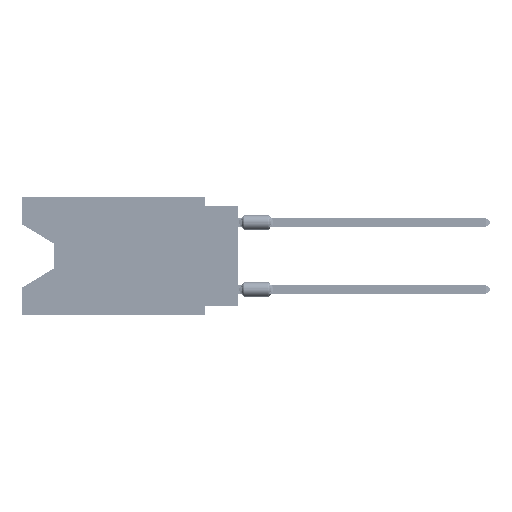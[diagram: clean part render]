
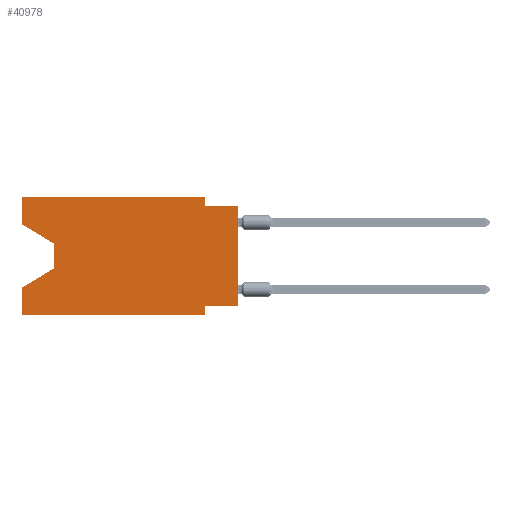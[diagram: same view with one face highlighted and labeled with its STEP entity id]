
A CAD part, left-side view. The second image highlights one B-rep face of the part: STEP entity #40978.
In plain terms, the highlighted planar face has unit normal (-1, 0, 0).
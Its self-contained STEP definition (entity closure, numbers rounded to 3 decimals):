
#410 = EDGE_CURVE ( 'NONE', #22969, #66952, #97227, .T. ) ;
#1054 = DIRECTION ( 'NONE',  ( 0., 0., -1. ) ) ;
#1590 = LINE ( 'NONE', #68167, #106151 ) ;
#3499 = ORIENTED_EDGE ( 'NONE', *, *, #56066, .T. ) ;
#3960 = DIRECTION ( 'NONE',  ( 0., 0., -1. ) ) ;
#5031 = PLANE ( 'NONE',  #49814 ) ;
#7524 = CARTESIAN_POINT ( 'NONE',  ( 0., 2.54, -0.635 ) ) ;
#9177 = VERTEX_POINT ( 'NONE', #7524 ) ;
#12287 = CARTESIAN_POINT ( 'NONE',  ( 0., 13.97, -3.505 ) ) ;
#13808 = CARTESIAN_POINT ( 'NONE',  ( 0., 2.54, -8.255 ) ) ;
#14338 = DIRECTION ( 'NONE',  ( 0., 0.855, -0.519 ) ) ;
#14988 = CARTESIAN_POINT ( 'NONE',  ( 0., 2.54, 0. ) ) ;
#15196 = VERTEX_POINT ( 'NONE', #34974 ) ;
#17138 = DIRECTION ( 'NONE',  ( 0., 0., 1. ) ) ;
#17782 = DIRECTION ( 'NONE',  ( 0., 0., 1. ) ) ;
#19921 = ORIENTED_EDGE ( 'NONE', *, *, #41716, .F. ) ;
#20324 = FACE_OUTER_BOUND ( 'NONE', #63549, .T. ) ;
#22209 = EDGE_CURVE ( 'NONE', #15196, #106065, #46941, .T. ) ;
#22969 = VERTEX_POINT ( 'NONE', #81820 ) ;
#23919 = DIRECTION ( 'NONE',  ( 0., -1., 0. ) ) ;
#24839 = EDGE_CURVE ( 'NONE', #106065, #89694, #95804, .T. ) ;
#25006 = LINE ( 'NONE', #98647, #97730 ) ;
#25774 = ORIENTED_EDGE ( 'NONE', *, *, #36053, .T. ) ;
#27647 = DIRECTION ( 'NONE',  ( 0., -1., 0. ) ) ;
#28692 = VERTEX_POINT ( 'NONE', #44951 ) ;
#29619 = CARTESIAN_POINT ( 'NONE',  ( 0., 16.383, 0. ) ) ;
#29656 = CARTESIAN_POINT ( 'NONE',  ( 0., 13.97, -3.505 ) ) ;
#29750 = DIRECTION ( 'NONE',  ( 0., 0., -1. ) ) ;
#30742 = VECTOR ( 'NONE', #96282, 1000. ) ;
#31433 = EDGE_CURVE ( 'NONE', #15196, #68803, #40127, .T. ) ;
#34974 = CARTESIAN_POINT ( 'NONE',  ( 0., 16.383, -2.038 ) ) ;
#36053 = EDGE_CURVE ( 'NONE', #95452, #57913, #43953, .T. ) ;
#36212 = EDGE_CURVE ( 'NONE', #68803, #22969, #62446, .T. ) ;
#36391 = VECTOR ( 'NONE', #82103, 1000. ) ;
#36546 = VECTOR ( 'NONE', #27647, 1000. ) ;
#40127 = LINE ( 'NONE', #89203, #36391 ) ;
#40978 = ADVANCED_FACE ( 'NONE', ( #20324 ), #5031, .F. ) ;
#41714 = CARTESIAN_POINT ( 'NONE',  ( 0., 16.383, 0. ) ) ;
#41716 = EDGE_CURVE ( 'NONE', #89694, #9177, #45599, .T. ) ;
#42462 = DIRECTION ( 'NONE',  ( 0., -1., 0. ) ) ;
#42881 = CARTESIAN_POINT ( 'NONE',  ( 0., 16.383, -6.852 ) ) ;
#43953 = LINE ( 'NONE', #101233, #91991 ) ;
#44951 = CARTESIAN_POINT ( 'NONE',  ( 0., 2.54, -8.89 ) ) ;
#45599 = LINE ( 'NONE', #55347, #30742 ) ;
#45636 = ORIENTED_EDGE ( 'NONE', *, *, #78767, .F. ) ;
#46403 = DIRECTION ( 'NONE',  ( 0., 0., 1. ) ) ;
#46941 = LINE ( 'NONE', #89463, #76501 ) ;
#49564 = CARTESIAN_POINT ( 'NONE',  ( 0., 0., -0.635 ) ) ;
#49814 = AXIS2_PLACEMENT_3D ( 'NONE', #29619, #86869, #3960 ) ;
#50976 = CARTESIAN_POINT ( 'NONE',  ( 0., 16.383, 0. ) ) ;
#53690 = VECTOR ( 'NONE', #42462, 1000. ) ;
#54355 = CARTESIAN_POINT ( 'NONE',  ( 0., 16.383, 0. ) ) ;
#54443 = EDGE_CURVE ( 'NONE', #89322, #28692, #1590, .T. ) ;
#55347 = CARTESIAN_POINT ( 'NONE',  ( 0., 2.54, 0. ) ) ;
#55405 = VECTOR ( 'NONE', #29750, 1000. ) ;
#55783 = CARTESIAN_POINT ( 'NONE',  ( 0., 13.97, -5.385 ) ) ;
#56066 = EDGE_CURVE ( 'NONE', #106094, #28692, #25006, .T. ) ;
#57913 = VERTEX_POINT ( 'NONE', #104447 ) ;
#60209 = CARTESIAN_POINT ( 'NONE',  ( 0., 16.383, -8.89 ) ) ;
#62446 = LINE ( 'NONE', #12287, #55405 ) ;
#63549 = EDGE_LOOP ( 'NONE', ( #106883, #97300, #88771, #93473, #3499, #90424, #45636, #25774, #83132, #19921, #72074, #102003 ) ) ;
#65926 = LINE ( 'NONE', #49564, #53690 ) ;
#66952 = VERTEX_POINT ( 'NONE', #42881 ) ;
#68167 = CARTESIAN_POINT ( 'NONE',  ( 0., 2.54, -8.89 ) ) ;
#68803 = VERTEX_POINT ( 'NONE', #29656 ) ;
#68848 = VECTOR ( 'NONE', #17138, 1000. ) ;
#72074 = ORIENTED_EDGE ( 'NONE', *, *, #24839, .F. ) ;
#73374 = LINE ( 'NONE', #41714, #68848 ) ;
#76501 = VECTOR ( 'NONE', #46403, 1000. ) ;
#78767 = EDGE_CURVE ( 'NONE', #95452, #89322, #94426, .T. ) ;
#81820 = CARTESIAN_POINT ( 'NONE',  ( 0., 13.97, -5.385 ) ) ;
#82103 = DIRECTION ( 'NONE',  ( 0., -0.855, -0.519 ) ) ;
#83132 = ORIENTED_EDGE ( 'NONE', *, *, #90288, .F. ) ;
#83478 = CARTESIAN_POINT ( 'NONE',  ( 0., 0., -8.255 ) ) ;
#86152 = VECTOR ( 'NONE', #94946, 1000. ) ;
#86869 = DIRECTION ( 'NONE',  ( 1., 0., 0. ) ) ;
#88771 = ORIENTED_EDGE ( 'NONE', *, *, #410, .T. ) ;
#89203 = CARTESIAN_POINT ( 'NONE',  ( 0., 16.383, -2.038 ) ) ;
#89322 = VERTEX_POINT ( 'NONE', #13808 ) ;
#89463 = CARTESIAN_POINT ( 'NONE',  ( 0., 16.383, 0. ) ) ;
#89694 = VERTEX_POINT ( 'NONE', #14988 ) ;
#90288 = EDGE_CURVE ( 'NONE', #9177, #57913, #65926, .T. ) ;
#90424 = ORIENTED_EDGE ( 'NONE', *, *, #54443, .F. ) ;
#91991 = VECTOR ( 'NONE', #17782, 1000. ) ;
#93473 = ORIENTED_EDGE ( 'NONE', *, *, #100284, .F. ) ;
#94426 = LINE ( 'NONE', #102600, #86152 ) ;
#94946 = DIRECTION ( 'NONE',  ( 0., 1., 0. ) ) ;
#95452 = VERTEX_POINT ( 'NONE', #83478 ) ;
#95804 = LINE ( 'NONE', #54355, #36546 ) ;
#96282 = DIRECTION ( 'NONE',  ( 0., 0., -1. ) ) ;
#97227 = LINE ( 'NONE', #55783, #98364 ) ;
#97300 = ORIENTED_EDGE ( 'NONE', *, *, #36212, .T. ) ;
#97730 = VECTOR ( 'NONE', #23919, 1000. ) ;
#98364 = VECTOR ( 'NONE', #14338, 1000. ) ;
#98647 = CARTESIAN_POINT ( 'NONE',  ( 0., 16.383, -8.89 ) ) ;
#100284 = EDGE_CURVE ( 'NONE', #106094, #66952, #73374, .T. ) ;
#101233 = CARTESIAN_POINT ( 'NONE',  ( 0., 0., 0. ) ) ;
#102003 = ORIENTED_EDGE ( 'NONE', *, *, #22209, .F. ) ;
#102600 = CARTESIAN_POINT ( 'NONE',  ( 0., 0., -8.255 ) ) ;
#104447 = CARTESIAN_POINT ( 'NONE',  ( 0., 0., -0.635 ) ) ;
#106065 = VERTEX_POINT ( 'NONE', #50976 ) ;
#106094 = VERTEX_POINT ( 'NONE', #60209 ) ;
#106151 = VECTOR ( 'NONE', #1054, 1000. ) ;
#106883 = ORIENTED_EDGE ( 'NONE', *, *, #31433, .T. ) ;
